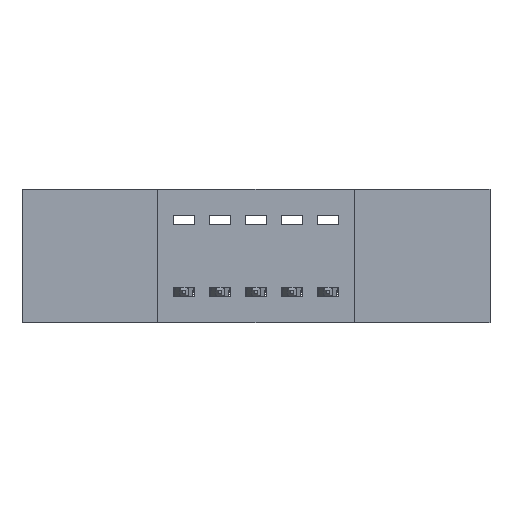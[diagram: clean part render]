
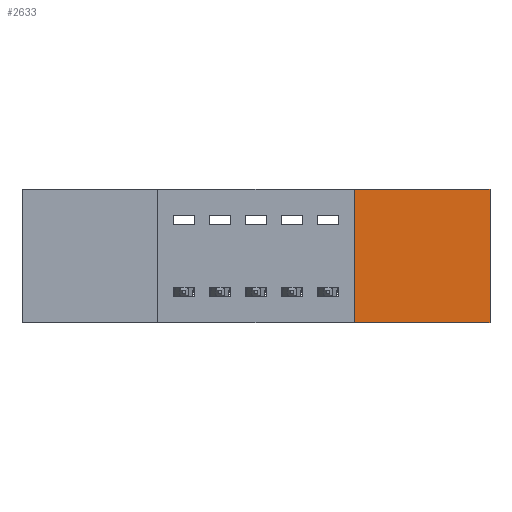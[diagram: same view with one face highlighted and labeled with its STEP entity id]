
A CAD part, front view. The second image highlights one B-rep face of the part: STEP entity #2633.
In plain terms, the highlighted planar face has unit normal (0, -1, 0).
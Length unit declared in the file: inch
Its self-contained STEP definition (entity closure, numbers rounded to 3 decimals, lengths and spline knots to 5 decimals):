
#57 = VECTOR ( 'NONE', #1124, 39.37008 ) ;
#133 = EDGE_LOOP ( 'NONE', ( #190, #2595, #2405, #756 ) ) ;
#190 = ORIENTED_EDGE ( 'NONE', *, *, #4661, .F. ) ;
#359 = LINE ( 'NONE', #2389, #7546 ) ;
#756 = ORIENTED_EDGE ( 'NONE', *, *, #3116, .F. ) ;
#869 = VECTOR ( 'NONE', #1510, 39.37008 ) ;
#1124 = DIRECTION ( 'NONE',  ( -1., 0., 0. ) ) ;
#1138 = VECTOR ( 'NONE', #5217, 39.37008 ) ;
#1176 = DIRECTION ( 'NONE',  ( 0., 0., -1. ) ) ;
#1198 = DIRECTION ( 'NONE',  ( 0., -1., 0. ) ) ;
#1337 = VERTEX_POINT ( 'NONE', #7448 ) ;
#1510 = DIRECTION ( 'NONE',  ( 1., 0., 0. ) ) ;
#1671 = VERTEX_POINT ( 'NONE', #5889 ) ;
#2389 = CARTESIAN_POINT ( 'NONE',  ( 1.3, 0., 0. ) ) ;
#2405 = ORIENTED_EDGE ( 'NONE', *, *, #5117, .F. ) ;
#2595 = ORIENTED_EDGE ( 'NONE', *, *, #5752, .F. ) ;
#2633 = ADVANCED_FACE ( 'NONE', ( #4340 ), #5917, .T. ) ;
#2796 = CARTESIAN_POINT ( 'NONE',  ( 0., 0., -0.37 ) ) ;
#3116 = EDGE_CURVE ( 'NONE', #5296, #4411, #3954, .T. ) ;
#3272 = AXIS2_PLACEMENT_3D ( 'NONE', #5949, #1198, #1176 ) ;
#3332 = LINE ( 'NONE', #2796, #57 ) ;
#3954 = LINE ( 'NONE', #4289, #869 ) ;
#4289 = CARTESIAN_POINT ( 'NONE',  ( 0., 0., 0. ) ) ;
#4340 = FACE_OUTER_BOUND ( 'NONE', #133, .T. ) ;
#4411 = VERTEX_POINT ( 'NONE', #4473 ) ;
#4473 = CARTESIAN_POINT ( 'NONE',  ( 1.3, 0., 0. ) ) ;
#4661 = EDGE_CURVE ( 'NONE', #1337, #5296, #7462, .T. ) ;
#4750 = CARTESIAN_POINT ( 'NONE',  ( 0.923, 0., -0.37 ) ) ;
#4850 = CARTESIAN_POINT ( 'NONE',  ( 0.923, 0., 0. ) ) ;
#5117 = EDGE_CURVE ( 'NONE', #4411, #1671, #359, .T. ) ;
#5217 = DIRECTION ( 'NONE',  ( 0., 0., 1. ) ) ;
#5296 = VERTEX_POINT ( 'NONE', #4850 ) ;
#5752 = EDGE_CURVE ( 'NONE', #1671, #1337, #3332, .T. ) ;
#5889 = CARTESIAN_POINT ( 'NONE',  ( 1.3, 0., -0.37 ) ) ;
#5917 = PLANE ( 'NONE',  #3272 ) ;
#5949 = CARTESIAN_POINT ( 'NONE',  ( 0., 0., -0.37 ) ) ;
#7099 = DIRECTION ( 'NONE',  ( 0., 0., -1. ) ) ;
#7448 = CARTESIAN_POINT ( 'NONE',  ( 0.923, 0., -0.37 ) ) ;
#7462 = LINE ( 'NONE', #4750, #1138 ) ;
#7546 = VECTOR ( 'NONE', #7099, 39.37008 ) ;
